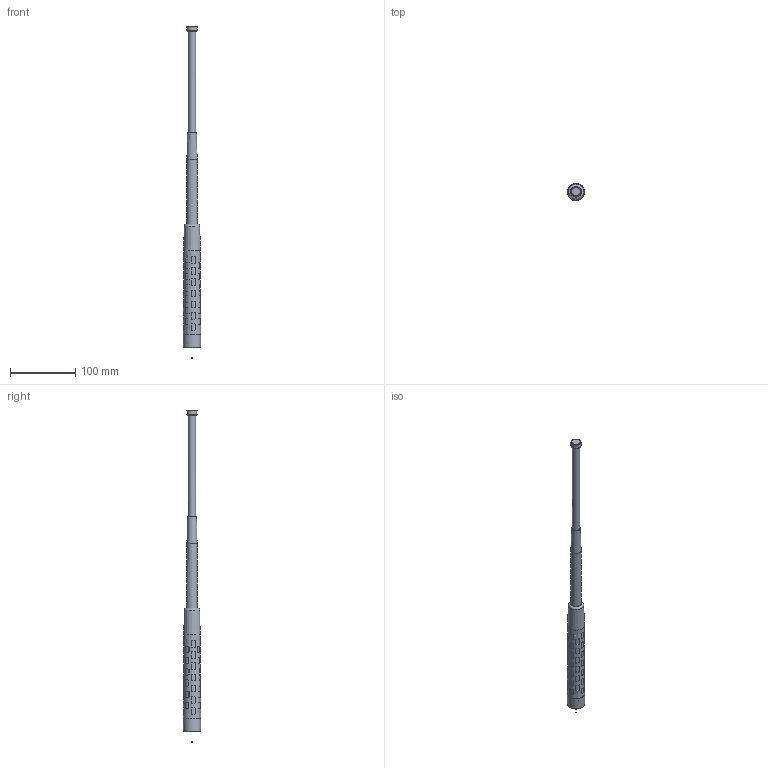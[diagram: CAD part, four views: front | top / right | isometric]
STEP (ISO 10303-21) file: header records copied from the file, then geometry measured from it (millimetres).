
FILE_DESCRIPTION(('STEP AP214'),'1');
FILE_NAME('schlagstock.stp','2020-11-01T12:06:00',(' '),(' '),'Spatial InterOp 3D',' ',' ');
FILE_SCHEMA(('AUTOMOTIVE_DESIGN { 1 0 10303 214 1 1 1 1 }'));
Length unit declared in the file: metre
Products named in the file (6): 1604304569; 1604300746; 1604300735; 1604221803; 1604218462; 1604218398
Bounding box: 26.49 x 26.48 x 510.49 mm (x, y, z)
Volume: 81635.9 mm3; surface area: 56967.8 mm2
Topology: 6 solids, 6 shells, 303 faces, 725 edges, 483 vertices
Faces by surface type: plane 218, cone 62, cylinder 8, torus 8, bspline 7
Full cylindrical faces by diameter (mm): 8 x1, 8.2 x1, 11.3 x1, 20.7 x1, 20.8 x1, 23.9 x1, 24 x1, 26.5 x1
Entity records: 11265 total; most frequent: CARTESIAN_POINT 2160, ORIENTED_EDGE 1332, DIRECTION 1314, EDGE_CURVE 666, AXIS2_PLACEMENT_3D 549, VERTEX_POINT 457, EDGE_LOOP 391, FACE_OUTER_BOUND 319
